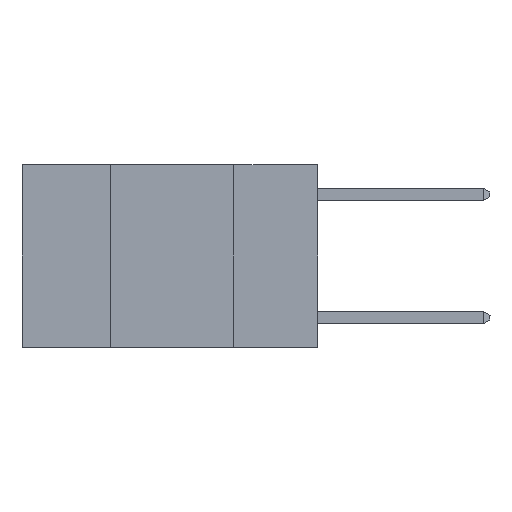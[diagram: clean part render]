
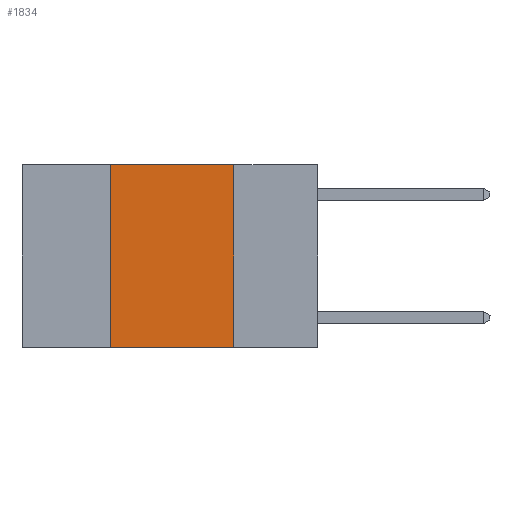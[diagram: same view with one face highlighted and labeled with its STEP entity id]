
A CAD part, left-side view. The second image highlights one B-rep face of the part: STEP entity #1834.
In plain terms, the highlighted planar face has unit normal (-1, 0, 0).
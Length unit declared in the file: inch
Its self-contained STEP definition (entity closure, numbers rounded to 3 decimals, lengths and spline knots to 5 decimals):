
#575 = VECTOR ( 'NONE', #1551, 39.37008 ) ;
#1082 = LINE ( 'NONE', #3588, #575 ) ;
#1377 = CARTESIAN_POINT ( 'NONE',  ( 0., 0.17, -0.37 ) ) ;
#1551 = DIRECTION ( 'NONE',  ( 0., -1., 0. ) ) ;
#1834 = ADVANCED_FACE ( 'NONE', ( #5928 ), #2035, .F. ) ;
#2035 = PLANE ( 'NONE',  #4635 ) ;
#2255 = VERTEX_POINT ( 'NONE', #2671 ) ;
#2671 = CARTESIAN_POINT ( 'NONE',  ( 0., 0.42, -0.37 ) ) ;
#2781 = CARTESIAN_POINT ( 'NONE',  ( 0., 0.17, 0. ) ) ;
#2833 = DIRECTION ( 'NONE',  ( 0., 0., -1. ) ) ;
#3406 = DIRECTION ( 'NONE',  ( 0., 0., -1. ) ) ;
#3488 = EDGE_CURVE ( 'NONE', #5867, #5671, #4543, .T. ) ;
#3588 = CARTESIAN_POINT ( 'NONE',  ( 0., 0.6, 0. ) ) ;
#3620 = ORIENTED_EDGE ( 'NONE', *, *, #4006, .F. ) ;
#4006 = EDGE_CURVE ( 'NONE', #2255, #7704, #7929, .T. ) ;
#4065 = EDGE_CURVE ( 'NONE', #7704, #5867, #1082, .T. ) ;
#4182 = EDGE_LOOP ( 'NONE', ( #6197, #8224, #3620, #7978 ) ) ;
#4389 = VECTOR ( 'NONE', #2833, 39.37008 ) ;
#4543 = LINE ( 'NONE', #6637, #4389 ) ;
#4603 = CARTESIAN_POINT ( 'NONE',  ( 0., 0.42, 0. ) ) ;
#4615 = EDGE_CURVE ( 'NONE', #2255, #5671, #6238, .T. ) ;
#4622 = DIRECTION ( 'NONE',  ( 1., 0., 0. ) ) ;
#4635 = AXIS2_PLACEMENT_3D ( 'NONE', #6608, #4622, #3406 ) ;
#4797 = VECTOR ( 'NONE', #5559, 39.37008 ) ;
#4923 = CARTESIAN_POINT ( 'NONE',  ( 0., 0.42, 0. ) ) ;
#5187 = VECTOR ( 'NONE', #6666, 39.37008 ) ;
#5559 = DIRECTION ( 'NONE',  ( 0., -1., 0. ) ) ;
#5671 = VERTEX_POINT ( 'NONE', #1377 ) ;
#5867 = VERTEX_POINT ( 'NONE', #2781 ) ;
#5928 = FACE_OUTER_BOUND ( 'NONE', #4182, .T. ) ;
#6197 = ORIENTED_EDGE ( 'NONE', *, *, #3488, .F. ) ;
#6238 = LINE ( 'NONE', #6317, #4797 ) ;
#6317 = CARTESIAN_POINT ( 'NONE',  ( 0., 0.6, -0.37 ) ) ;
#6608 = CARTESIAN_POINT ( 'NONE',  ( 0., 0.6, 0. ) ) ;
#6637 = CARTESIAN_POINT ( 'NONE',  ( 0., 0.17, 0. ) ) ;
#6666 = DIRECTION ( 'NONE',  ( 0., 0., 1. ) ) ;
#7704 = VERTEX_POINT ( 'NONE', #4923 ) ;
#7929 = LINE ( 'NONE', #4603, #5187 ) ;
#7978 = ORIENTED_EDGE ( 'NONE', *, *, #4615, .T. ) ;
#8224 = ORIENTED_EDGE ( 'NONE', *, *, #4065, .F. ) ;
